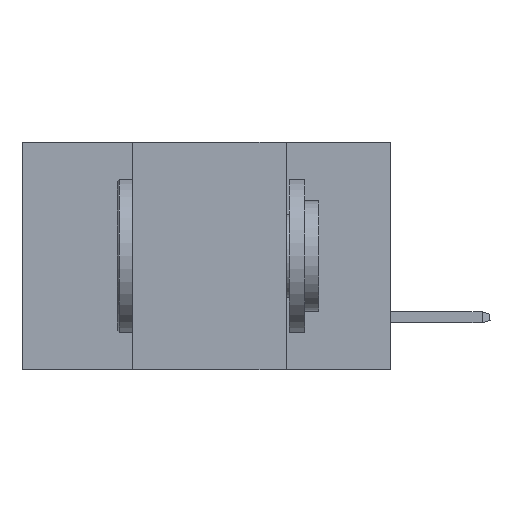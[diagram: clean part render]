
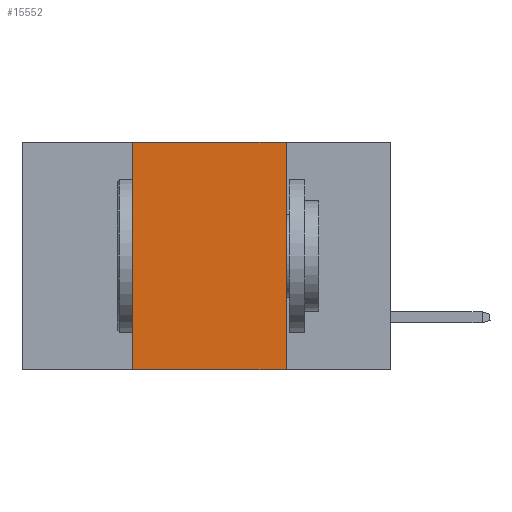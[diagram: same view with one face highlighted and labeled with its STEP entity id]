
A CAD part, left-side view. The second image highlights one B-rep face of the part: STEP entity #15552.
In plain terms, the highlighted planar face has unit normal (-1, 0, 0).
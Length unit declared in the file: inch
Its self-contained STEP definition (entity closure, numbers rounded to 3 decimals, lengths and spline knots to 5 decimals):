
#1183 = FACE_OUTER_BOUND ( 'NONE', #2306, .T. ) ;
#2306 = EDGE_LOOP ( 'NONE', ( #12359, #48483, #23913, #38549 ) ) ;
#4556 = DIRECTION ( 'NONE',  ( 0., 0., 1. ) ) ;
#6019 = DIRECTION ( 'NONE',  ( 0., -1., 0. ) ) ;
#8846 = CARTESIAN_POINT ( 'NONE',  ( 0., 0.17, -0.37 ) ) ;
#9054 = VERTEX_POINT ( 'NONE', #14649 ) ;
#9179 = LINE ( 'NONE', #23433, #44957 ) ;
#10758 = DIRECTION ( 'NONE',  ( 0., 0., -1. ) ) ;
#12359 = ORIENTED_EDGE ( 'NONE', *, *, #48717, .F. ) ;
#12420 = LINE ( 'NONE', #31031, #18996 ) ;
#13454 = EDGE_CURVE ( 'NONE', #9054, #17583, #38279, .T. ) ;
#13712 = VECTOR ( 'NONE', #10758, 39.37008 ) ;
#14649 = CARTESIAN_POINT ( 'NONE',  ( 0., 0.42, -0.37 ) ) ;
#15552 = ADVANCED_FACE ( 'NONE', ( #1183 ), #25016, .F. ) ;
#17583 = VERTEX_POINT ( 'NONE', #8846 ) ;
#18197 = CARTESIAN_POINT ( 'NONE',  ( 0., 0.17, 0. ) ) ;
#18883 = VERTEX_POINT ( 'NONE', #20736 ) ;
#18996 = VECTOR ( 'NONE', #39488, 39.37008 ) ;
#20736 = CARTESIAN_POINT ( 'NONE',  ( 0., 0.17, 0. ) ) ;
#21304 = CARTESIAN_POINT ( 'NONE',  ( 0., 0.42, 0. ) ) ;
#23433 = CARTESIAN_POINT ( 'NONE',  ( 0., 0.42, 0. ) ) ;
#23913 = ORIENTED_EDGE ( 'NONE', *, *, #46077, .F. ) ;
#25016 = PLANE ( 'NONE',  #43419 ) ;
#25018 = LINE ( 'NONE', #18197, #13712 ) ;
#25309 = EDGE_CURVE ( 'NONE', #32846, #18883, #12420, .T. ) ;
#28197 = VECTOR ( 'NONE', #6019, 39.37008 ) ;
#31031 = CARTESIAN_POINT ( 'NONE',  ( 0., 0.6, 0. ) ) ;
#32149 = DIRECTION ( 'NONE',  ( 1., 0., 0. ) ) ;
#32846 = VERTEX_POINT ( 'NONE', #21304 ) ;
#32941 = CARTESIAN_POINT ( 'NONE',  ( 0., 0.6, -0.37 ) ) ;
#38279 = LINE ( 'NONE', #32941, #28197 ) ;
#38549 = ORIENTED_EDGE ( 'NONE', *, *, #13454, .T. ) ;
#39488 = DIRECTION ( 'NONE',  ( 0., -1., 0. ) ) ;
#41152 = DIRECTION ( 'NONE',  ( 0., 0., -1. ) ) ;
#43419 = AXIS2_PLACEMENT_3D ( 'NONE', #47223, #32149, #41152 ) ;
#44957 = VECTOR ( 'NONE', #4556, 39.37008 ) ;
#46077 = EDGE_CURVE ( 'NONE', #9054, #32846, #9179, .T. ) ;
#47223 = CARTESIAN_POINT ( 'NONE',  ( 0., 0.6, 0. ) ) ;
#48483 = ORIENTED_EDGE ( 'NONE', *, *, #25309, .F. ) ;
#48717 = EDGE_CURVE ( 'NONE', #18883, #17583, #25018, .T. ) ;
